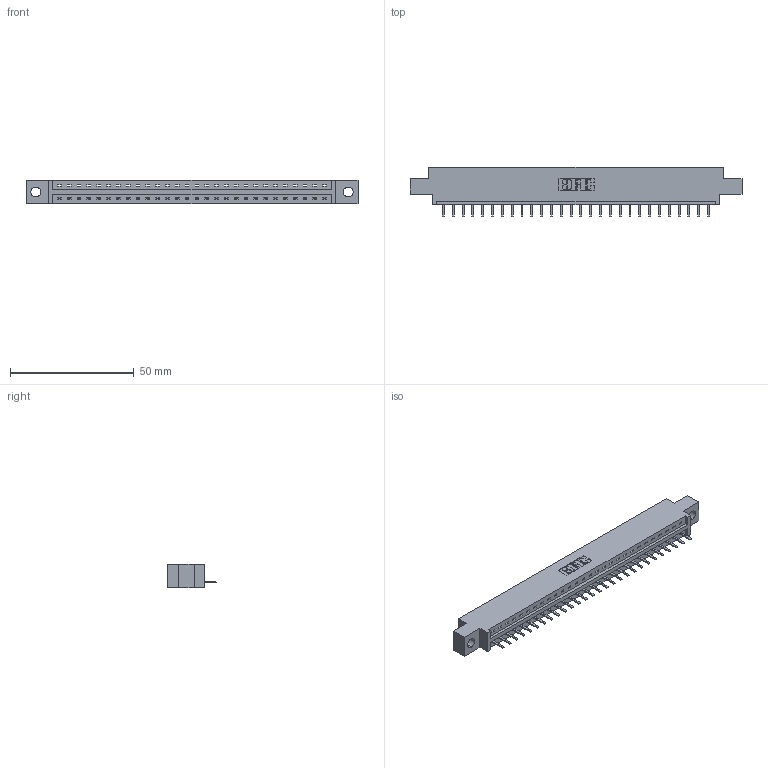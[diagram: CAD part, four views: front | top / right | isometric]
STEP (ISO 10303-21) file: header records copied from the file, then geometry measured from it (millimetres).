
FILE_DESCRIPTION (( 'STEP AP203' ), '1' );
FILE_NAME ('387-028-520-604.STEP', '2019-10-03T14:33:51', ( '' ), ( '' ), 'SwSTEP 2.0', 'SolidWorks 2016', '' );
FILE_SCHEMA (( 'CONFIG_CONTROL_DESIGN' ));
Length unit declared in the file: inch
Products named in the file (3): 337 Part_0.170 Offset - 0.156 Dia-TH; 387-028-520-604; 345-292-001_345-293-120
Assembly tree (29 placements, depth 2):
  387-028-520-604
    337 Part_0.170 Offset - 0.156 Dia-TH
    345-292-001_345-293-120  x28
Bounding box: 133.96 x 20.02 x 9.4 mm (x, y, z)
Volume: 13461.8 mm3; surface area: 13434.8 mm2
Topology: 29 solids, 29 shells, 1966 faces, 5811 edges, 3798 vertices
Faces by surface type: plane 1418, cylinder 548
Entity records: 22873 total; most frequent: CARTESIAN_POINT 4002, ORIENTED_EDGE 3954, DIRECTION 3385, EDGE_CURVE 1977, LINE 1845, VECTOR 1845, VERTEX_POINT 1314, AXIS2_PLACEMENT_3D 770
